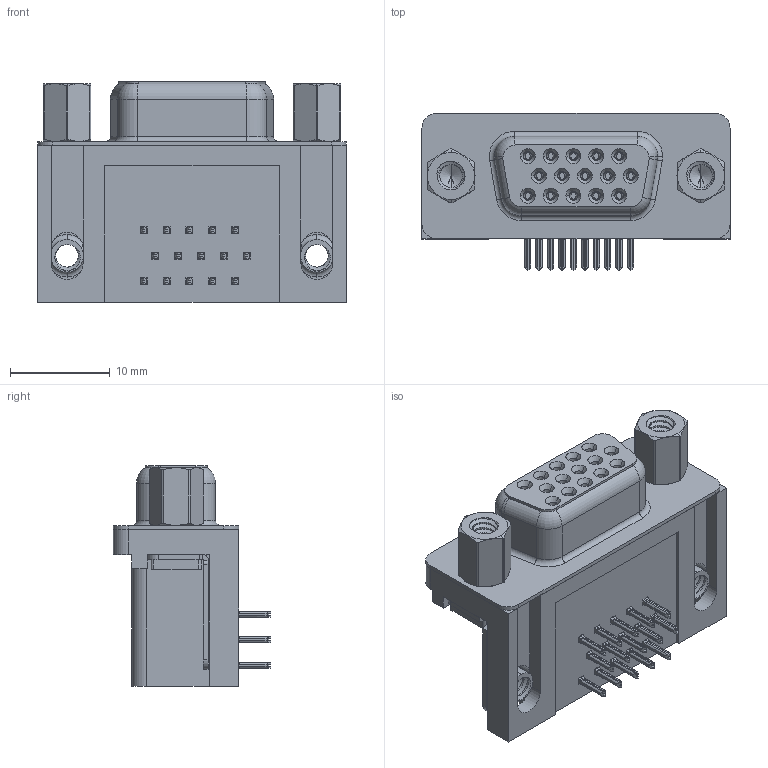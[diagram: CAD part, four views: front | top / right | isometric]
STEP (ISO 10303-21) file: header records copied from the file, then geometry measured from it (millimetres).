
FILE_DESCRIPTION (( 'STEP AP203' ), '1' );
FILE_NAME ('634-015-674-053.STEP', '2018-11-09T22:53:01', ( '' ), ( '' ), 'SwSTEP 2.0', 'SolidWorks 2016', '' );
FILE_SCHEMA (( 'CONFIG_CONTROL_DESIGN' ));
Length unit declared in the file: millimetre
Products named in the file (10): 4-40 Threaded Rivet; 4-40 Hex Standoff; 634 Housing; 634-015-674-053; 634 Shell; Contact Bottom; Contact Middle; Contact Top; 4-40 Threaded Board Mount; Contact Middle_Recessed
Assembly tree (23 placements, depth 2):
  634-015-674-053
    634 Housing
    634 Shell
    Contact Bottom  x5
    Contact Middle  x4
    Contact Top  x5
    4-40 Threaded Board Mount  x2
    Contact Middle_Recessed
    4-40 Threaded Rivet  x2
    4-40 Hex Standoff  x2
Bounding box: 30.89 x 15.73 x 22.1 mm (x, y, z)
Volume: 4767 mm3; surface area: 7031.2 mm2
Topology: 23 solids, 23 shells, 2571 faces, 6774 edges, 4268 vertices
Faces by surface type: plane 1088, cylinder 675, bspline 544, cone 214, torus 50
Entity records: 43251 total; most frequent: CARTESIAN_POINT 18250, ORIENTED_EDGE 5302, DIRECTION 4299, EDGE_CURVE 2651, VERTEX_POINT 1686, VECTOR 1505, LINE 1505, AXIS2_PLACEMENT_3D 1397
